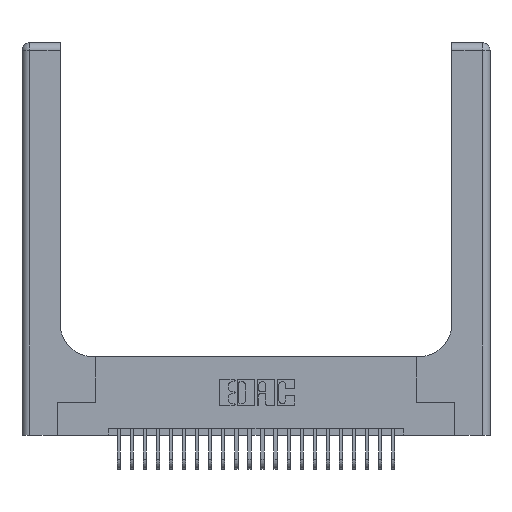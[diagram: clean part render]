
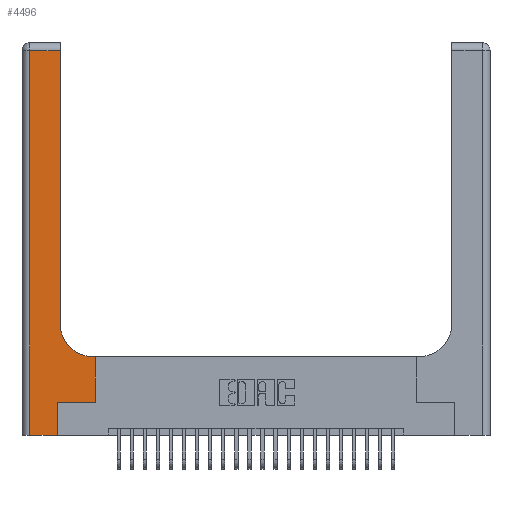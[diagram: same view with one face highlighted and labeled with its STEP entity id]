
A CAD part, top view. The second image highlights one B-rep face of the part: STEP entity #4496.
In plain terms, the highlighted planar face has unit normal (0, 0, 1).
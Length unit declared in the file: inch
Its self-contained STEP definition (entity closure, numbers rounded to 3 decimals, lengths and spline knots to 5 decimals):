
#125 = PLANE ( 'NONE',  #7126 ) ;
#603 = CARTESIAN_POINT ( 'NONE',  ( 0.2915, 2.94, 0.37 ) ) ;
#750 = DIRECTION ( 'NONE',  ( 0., 0., -1. ) ) ;
#1200 = LINE ( 'NONE', #17967, #15692 ) ;
#1231 = EDGE_CURVE ( 'NONE', #22027, #20500, #19124, .T. ) ;
#1856 = CARTESIAN_POINT ( 'NONE',  ( 0.269, 0., 0.37 ) ) ;
#2071 = DIRECTION ( 'NONE',  ( 0., 0., -1. ) ) ;
#2182 = ORIENTED_EDGE ( 'NONE', *, *, #1231, .T. ) ;
#2265 = LINE ( 'NONE', #14280, #7307 ) ;
#2804 = LINE ( 'NONE', #1856, #12836 ) ;
#3191 = VERTEX_POINT ( 'NONE', #9371 ) ;
#3547 = DIRECTION ( 'NONE',  ( -1., 0., 0. ) ) ;
#3631 = EDGE_CURVE ( 'NONE', #5948, #16330, #1200, .T. ) ;
#3894 = CARTESIAN_POINT ( 'NONE',  ( 0., 3., 0.37 ) ) ;
#4310 = CARTESIAN_POINT ( 'NONE',  ( 0.2915, 0.85, 0.37 ) ) ;
#4496 = ADVANCED_FACE ( 'NONE', ( #12715 ), #125, .F. ) ;
#4671 = ORIENTED_EDGE ( 'NONE', *, *, #11529, .T. ) ;
#5317 = ORIENTED_EDGE ( 'NONE', *, *, #3631, .T. ) ;
#5409 = EDGE_CURVE ( 'NONE', #18110, #5948, #7079, .T. ) ;
#5462 = LINE ( 'NONE', #23222, #9892 ) ;
#5725 = EDGE_CURVE ( 'NONE', #13911, #13454, #20655, .T. ) ;
#5948 = VERTEX_POINT ( 'NONE', #4310 ) ;
#5983 = VERTEX_POINT ( 'NONE', #23289 ) ;
#6019 = ORIENTED_EDGE ( 'NONE', *, *, #10370, .T. ) ;
#7079 = CIRCLE ( 'NONE', #21366, 0.25 ) ;
#7126 = AXIS2_PLACEMENT_3D ( 'NONE', #3894, #2071, #15280 ) ;
#7187 = CARTESIAN_POINT ( 'NONE',  ( 0.5415, 0.6, 0.37 ) ) ;
#7307 = VECTOR ( 'NONE', #16194, 39.37008 ) ;
#8057 = EDGE_CURVE ( 'NONE', #16330, #3191, #5462, .T. ) ;
#9367 = LINE ( 'NONE', #20223, #18765 ) ;
#9371 = CARTESIAN_POINT ( 'NONE',  ( 0.06, 2.94, 0.37 ) ) ;
#9384 = DIRECTION ( 'NONE',  ( 1., 0., 0. ) ) ;
#9631 = CARTESIAN_POINT ( 'NONE',  ( 0., 0., 0.37 ) ) ;
#9649 = EDGE_CURVE ( 'NONE', #13454, #5983, #9367, .T. ) ;
#9892 = VECTOR ( 'NONE', #13787, 39.37008 ) ;
#10370 = EDGE_CURVE ( 'NONE', #20500, #13911, #2804, .T. ) ;
#10599 = VECTOR ( 'NONE', #9384, 39.37008 ) ;
#10802 = DIRECTION ( 'NONE',  ( 0., 1., 0. ) ) ;
#11355 = ORIENTED_EDGE ( 'NONE', *, *, #9649, .T. ) ;
#11529 = EDGE_CURVE ( 'NONE', #5983, #18110, #21946, .T. ) ;
#12068 = CARTESIAN_POINT ( 'NONE',  ( 0.5415, 0.85, 0.37 ) ) ;
#12519 = CARTESIAN_POINT ( 'NONE',  ( 0.06, 0., 0.37 ) ) ;
#12715 = FACE_OUTER_BOUND ( 'NONE', #20711, .T. ) ;
#12836 = VECTOR ( 'NONE', #15067, 39.37008 ) ;
#12912 = ORIENTED_EDGE ( 'NONE', *, *, #15813, .T. ) ;
#13454 = VERTEX_POINT ( 'NONE', #16825 ) ;
#13787 = DIRECTION ( 'NONE',  ( -1., 0., 0. ) ) ;
#13911 = VERTEX_POINT ( 'NONE', #24485 ) ;
#13972 = DIRECTION ( 'NONE',  ( 1., 0., 0. ) ) ;
#14116 = VECTOR ( 'NONE', #15530, 39.37008 ) ;
#14280 = CARTESIAN_POINT ( 'NONE',  ( 0.06, 3., 0.37 ) ) ;
#15067 = DIRECTION ( 'NONE',  ( 0., 1., 0. ) ) ;
#15221 = ORIENTED_EDGE ( 'NONE', *, *, #5409, .T. ) ;
#15280 = DIRECTION ( 'NONE',  ( -1., 0., 0. ) ) ;
#15530 = DIRECTION ( 'NONE',  ( 1., 0., 0. ) ) ;
#15692 = VECTOR ( 'NONE', #16264, 39.37008 ) ;
#15813 = EDGE_CURVE ( 'NONE', #3191, #22027, #2265, .T. ) ;
#16194 = DIRECTION ( 'NONE',  ( 0., -1., 0. ) ) ;
#16264 = DIRECTION ( 'NONE',  ( 0., 1., 0. ) ) ;
#16330 = VERTEX_POINT ( 'NONE', #603 ) ;
#16742 = CARTESIAN_POINT ( 'NONE',  ( 0.2915, 0.6, 0.37 ) ) ;
#16825 = CARTESIAN_POINT ( 'NONE',  ( 0.5585, 0.25, 0.37 ) ) ;
#17967 = CARTESIAN_POINT ( 'NONE',  ( 0.2915, 3., 0.37 ) ) ;
#18085 = VECTOR ( 'NONE', #3547, 39.37008 ) ;
#18110 = VERTEX_POINT ( 'NONE', #7187 ) ;
#18745 = CARTESIAN_POINT ( 'NONE',  ( 0.269, 0.25, 0.37 ) ) ;
#18765 = VECTOR ( 'NONE', #10802, 39.37008 ) ;
#19124 = LINE ( 'NONE', #9631, #14116 ) ;
#20223 = CARTESIAN_POINT ( 'NONE',  ( 0.5585, 0.25, 0.37 ) ) ;
#20448 = CARTESIAN_POINT ( 'NONE',  ( 0.269, 0., 0.37 ) ) ;
#20500 = VERTEX_POINT ( 'NONE', #20448 ) ;
#20655 = LINE ( 'NONE', #18745, #10599 ) ;
#20709 = ORIENTED_EDGE ( 'NONE', *, *, #5725, .T. ) ;
#20711 = EDGE_LOOP ( 'NONE', ( #5317, #20791, #12912, #2182, #6019, #20709, #11355, #4671, #15221 ) ) ;
#20791 = ORIENTED_EDGE ( 'NONE', *, *, #8057, .T. ) ;
#21366 = AXIS2_PLACEMENT_3D ( 'NONE', #12068, #750, #13972 ) ;
#21946 = LINE ( 'NONE', #16742, #18085 ) ;
#22027 = VERTEX_POINT ( 'NONE', #12519 ) ;
#23222 = CARTESIAN_POINT ( 'NONE',  ( 0., 2.94, 0.37 ) ) ;
#23289 = CARTESIAN_POINT ( 'NONE',  ( 0.5585, 0.6, 0.37 ) ) ;
#24485 = CARTESIAN_POINT ( 'NONE',  ( 0.269, 0.25, 0.37 ) ) ;
